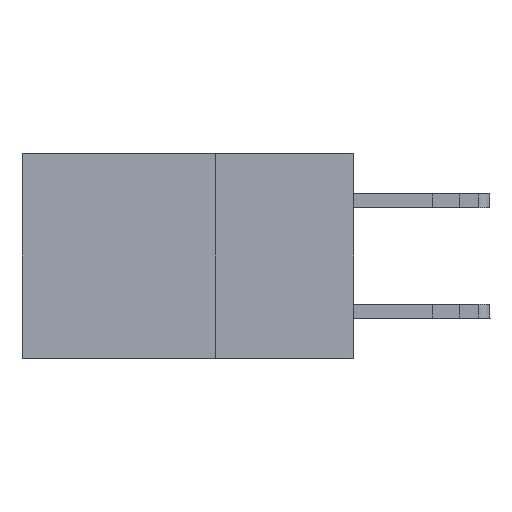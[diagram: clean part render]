
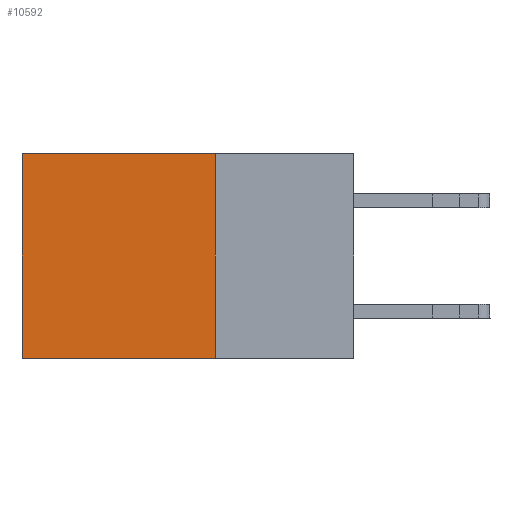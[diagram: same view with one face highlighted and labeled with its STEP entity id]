
A CAD part, left-side view. The second image highlights one B-rep face of the part: STEP entity #10592.
In plain terms, the highlighted planar face has unit normal (-1, 0, 0).
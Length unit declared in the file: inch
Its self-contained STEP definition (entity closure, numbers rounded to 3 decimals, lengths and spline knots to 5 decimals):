
#318 = LINE ( 'NONE', #7118, #7662 ) ;
#659 = LINE ( 'NONE', #3267, #15252 ) ;
#953 = VERTEX_POINT ( 'NONE', #8303 ) ;
#1922 = DIRECTION ( 'NONE',  ( 0., 1., 0. ) ) ;
#2152 = DIRECTION ( 'NONE',  ( 0., 0., -1. ) ) ;
#2847 = DIRECTION ( 'NONE',  ( 0., 0., -1. ) ) ;
#3267 = CARTESIAN_POINT ( 'NONE',  ( 0.2875, 0.25, 0. ) ) ;
#3487 = CARTESIAN_POINT ( 'NONE',  ( 0.2875, 0.25, 0. ) ) ;
#3611 = EDGE_CURVE ( 'NONE', #14672, #16382, #659, .T. ) ;
#4818 = VECTOR ( 'NONE', #12061, 39.37008 ) ;
#4888 = CARTESIAN_POINT ( 'NONE',  ( 0.2875, 0.25, -0.37 ) ) ;
#5176 = DIRECTION ( 'NONE',  ( 1., 0., 0. ) ) ;
#6057 = ORIENTED_EDGE ( 'NONE', *, *, #10504, .F. ) ;
#6380 = EDGE_CURVE ( 'NONE', #7135, #953, #7715, .T. ) ;
#7118 = CARTESIAN_POINT ( 'NONE',  ( 0.2875, 0.6, 0. ) ) ;
#7135 = VERTEX_POINT ( 'NONE', #8922 ) ;
#7363 = CARTESIAN_POINT ( 'NONE',  ( 0.2875, 0.6, 0. ) ) ;
#7662 = VECTOR ( 'NONE', #2847, 39.37008 ) ;
#7715 = LINE ( 'NONE', #4888, #4818 ) ;
#8216 = VECTOR ( 'NONE', #9014, 39.37008 ) ;
#8266 = CARTESIAN_POINT ( 'NONE',  ( 0.2875, 0.25, 0. ) ) ;
#8303 = CARTESIAN_POINT ( 'NONE',  ( 0.2875, 0.6, -0.37 ) ) ;
#8677 = ORIENTED_EDGE ( 'NONE', *, *, #3611, .T. ) ;
#8922 = CARTESIAN_POINT ( 'NONE',  ( 0.2875, 0.25, -0.37 ) ) ;
#8958 = ORIENTED_EDGE ( 'NONE', *, *, #13207, .T. ) ;
#9014 = DIRECTION ( 'NONE',  ( 0., 0., -1. ) ) ;
#10504 = EDGE_CURVE ( 'NONE', #14672, #7135, #10894, .T. ) ;
#10592 = ADVANCED_FACE ( 'NONE', ( #15849 ), #13676, .F. ) ;
#10894 = LINE ( 'NONE', #8266, #8216 ) ;
#12061 = DIRECTION ( 'NONE',  ( 0., 1., 0. ) ) ;
#12534 = EDGE_LOOP ( 'NONE', ( #8958, #15150, #6057, #8677 ) ) ;
#12539 = AXIS2_PLACEMENT_3D ( 'NONE', #3487, #5176, #2152 ) ;
#13207 = EDGE_CURVE ( 'NONE', #16382, #953, #318, .T. ) ;
#13237 = CARTESIAN_POINT ( 'NONE',  ( 0.2875, 0.25, 0. ) ) ;
#13676 = PLANE ( 'NONE',  #12539 ) ;
#14672 = VERTEX_POINT ( 'NONE', #13237 ) ;
#15150 = ORIENTED_EDGE ( 'NONE', *, *, #6380, .F. ) ;
#15252 = VECTOR ( 'NONE', #1922, 39.37008 ) ;
#15849 = FACE_OUTER_BOUND ( 'NONE', #12534, .T. ) ;
#16382 = VERTEX_POINT ( 'NONE', #7363 ) ;
